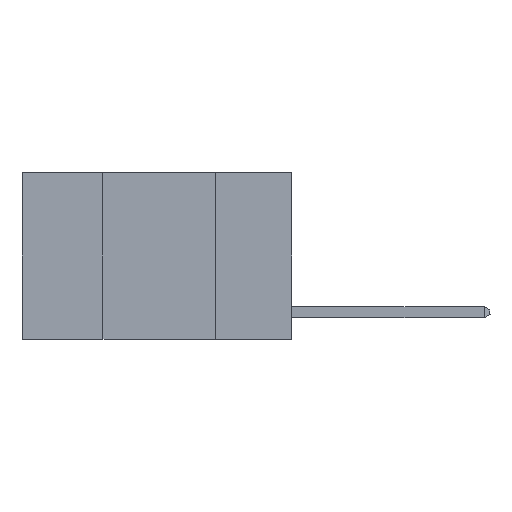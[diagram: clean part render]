
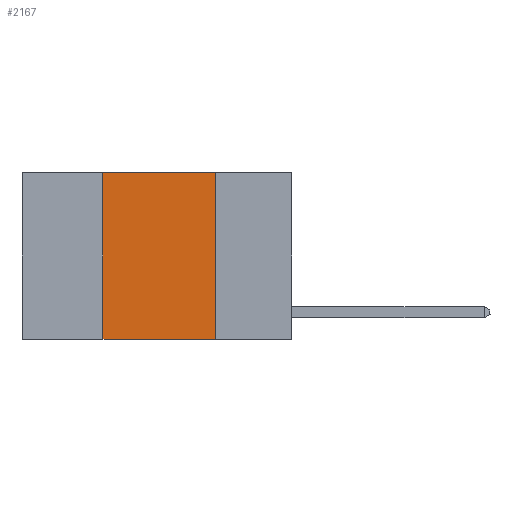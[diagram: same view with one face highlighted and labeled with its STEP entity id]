
A CAD part, left-side view. The second image highlights one B-rep face of the part: STEP entity #2167.
In plain terms, the highlighted planar face has unit normal (-1, 0, 0).
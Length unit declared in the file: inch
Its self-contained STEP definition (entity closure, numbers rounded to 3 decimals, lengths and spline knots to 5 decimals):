
#513 = EDGE_LOOP ( 'NONE', ( #10130, #4033, #7036, #1274 ) ) ;
#643 = CARTESIAN_POINT ( 'NONE',  ( 0., 0.6, 0. ) ) ;
#801 = CARTESIAN_POINT ( 'NONE',  ( 0., 0.42, -0.37 ) ) ;
#1029 = CARTESIAN_POINT ( 'NONE',  ( 0., 0.42, 0. ) ) ;
#1274 = ORIENTED_EDGE ( 'NONE', *, *, #3612, .T. ) ;
#1471 = VECTOR ( 'NONE', #7551, 39.37008 ) ;
#1627 = VERTEX_POINT ( 'NONE', #8531 ) ;
#1659 = DIRECTION ( 'NONE',  ( 0., -1., 0. ) ) ;
#2090 = DIRECTION ( 'NONE',  ( 0., 0., -1. ) ) ;
#2167 = ADVANCED_FACE ( 'NONE', ( #9993 ), #2205, .F. ) ;
#2205 = PLANE ( 'NONE',  #8480 ) ;
#2451 = LINE ( 'NONE', #9514, #1471 ) ;
#2491 = VERTEX_POINT ( 'NONE', #5351 ) ;
#2551 = CARTESIAN_POINT ( 'NONE',  ( 0., 0.6, -0.37 ) ) ;
#2558 = EDGE_CURVE ( 'NONE', #4005, #2491, #10524, .T. ) ;
#2968 = VECTOR ( 'NONE', #1659, 39.37008 ) ;
#3223 = VERTEX_POINT ( 'NONE', #8543 ) ;
#3612 = EDGE_CURVE ( 'NONE', #4005, #1627, #10264, .T. ) ;
#4005 = VERTEX_POINT ( 'NONE', #801 ) ;
#4033 = ORIENTED_EDGE ( 'NONE', *, *, #7238, .F. ) ;
#4447 = DIRECTION ( 'NONE',  ( 0., 0., 1. ) ) ;
#4614 = CARTESIAN_POINT ( 'NONE',  ( 0., 0.17, 0. ) ) ;
#4846 = DIRECTION ( 'NONE',  ( 0., 0., -1. ) ) ;
#5351 = CARTESIAN_POINT ( 'NONE',  ( 0., 0.42, 0. ) ) ;
#5598 = VECTOR ( 'NONE', #4447, 39.37008 ) ;
#5614 = DIRECTION ( 'NONE',  ( 1., 0., 0. ) ) ;
#6297 = LINE ( 'NONE', #4614, #6782 ) ;
#6782 = VECTOR ( 'NONE', #2090, 39.37008 ) ;
#7036 = ORIENTED_EDGE ( 'NONE', *, *, #2558, .F. ) ;
#7238 = EDGE_CURVE ( 'NONE', #2491, #3223, #2451, .T. ) ;
#7551 = DIRECTION ( 'NONE',  ( 0., -1., 0. ) ) ;
#8480 = AXIS2_PLACEMENT_3D ( 'NONE', #643, #5614, #4846 ) ;
#8531 = CARTESIAN_POINT ( 'NONE',  ( 0., 0.17, -0.37 ) ) ;
#8543 = CARTESIAN_POINT ( 'NONE',  ( 0., 0.17, 0. ) ) ;
#9514 = CARTESIAN_POINT ( 'NONE',  ( 0., 0.6, 0. ) ) ;
#9647 = EDGE_CURVE ( 'NONE', #3223, #1627, #6297, .T. ) ;
#9993 = FACE_OUTER_BOUND ( 'NONE', #513, .T. ) ;
#10130 = ORIENTED_EDGE ( 'NONE', *, *, #9647, .F. ) ;
#10264 = LINE ( 'NONE', #2551, #2968 ) ;
#10524 = LINE ( 'NONE', #1029, #5598 ) ;
